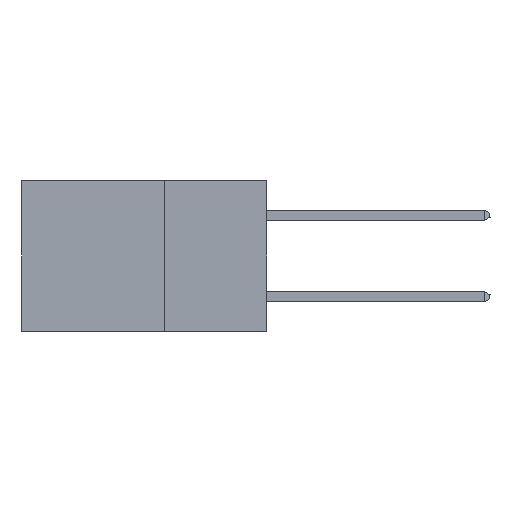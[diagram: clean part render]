
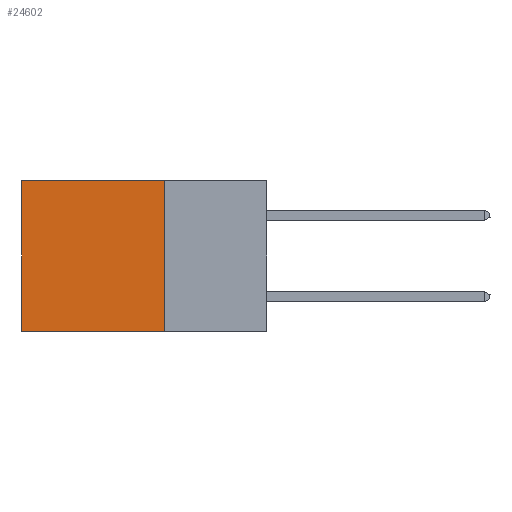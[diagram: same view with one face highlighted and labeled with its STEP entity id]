
A CAD part, left-side view. The second image highlights one B-rep face of the part: STEP entity #24602.
In plain terms, the highlighted planar face has unit normal (-1, 0, 0).
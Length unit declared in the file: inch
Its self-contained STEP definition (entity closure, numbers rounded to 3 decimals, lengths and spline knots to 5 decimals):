
#534 = EDGE_CURVE ( 'NONE', #13739, #16525, #32955, .T. ) ;
#2148 = DIRECTION ( 'NONE',  ( 0., 0., -1. ) ) ;
#2479 = DIRECTION ( 'NONE',  ( 0., 0., -1. ) ) ;
#3390 = DIRECTION ( 'NONE',  ( 0., 1., 0. ) ) ;
#8417 = CARTESIAN_POINT ( 'NONE',  ( 0.2875, 0.6, 0. ) ) ;
#9403 = AXIS2_PLACEMENT_3D ( 'NONE', #19149, #15584, #2479 ) ;
#9864 = EDGE_CURVE ( 'NONE', #23453, #16525, #13088, .T. ) ;
#10249 = CARTESIAN_POINT ( 'NONE',  ( 0.2875, 0.25, 0. ) ) ;
#10642 = VECTOR ( 'NONE', #12633, 39.37008 ) ;
#12633 = DIRECTION ( 'NONE',  ( 0., 1., 0. ) ) ;
#13088 = LINE ( 'NONE', #8417, #23168 ) ;
#13213 = EDGE_LOOP ( 'NONE', ( #23382, #16811, #35172, #29277 ) ) ;
#13739 = VERTEX_POINT ( 'NONE', #31877 ) ;
#14874 = EDGE_CURVE ( 'NONE', #38300, #23453, #29281, .T. ) ;
#15584 = DIRECTION ( 'NONE',  ( 1., 0., 0. ) ) ;
#16525 = VERTEX_POINT ( 'NONE', #26845 ) ;
#16811 = ORIENTED_EDGE ( 'NONE', *, *, #534, .F. ) ;
#19149 = CARTESIAN_POINT ( 'NONE',  ( 0.2875, 0.25, 0. ) ) ;
#21588 = VECTOR ( 'NONE', #22875, 39.37008 ) ;
#22875 = DIRECTION ( 'NONE',  ( 0., 0., -1. ) ) ;
#23168 = VECTOR ( 'NONE', #2148, 39.37008 ) ;
#23382 = ORIENTED_EDGE ( 'NONE', *, *, #9864, .T. ) ;
#23453 = VERTEX_POINT ( 'NONE', #36629 ) ;
#24602 = ADVANCED_FACE ( 'NONE', ( #30479 ), #33254, .F. ) ;
#26845 = CARTESIAN_POINT ( 'NONE',  ( 0.2875, 0.6, -0.37 ) ) ;
#26944 = EDGE_CURVE ( 'NONE', #38300, #13739, #32287, .T. ) ;
#29277 = ORIENTED_EDGE ( 'NONE', *, *, #14874, .T. ) ;
#29281 = LINE ( 'NONE', #40850, #30834 ) ;
#30479 = FACE_OUTER_BOUND ( 'NONE', #13213, .T. ) ;
#30744 = CARTESIAN_POINT ( 'NONE',  ( 0.2875, 0.25, -0.37 ) ) ;
#30834 = VECTOR ( 'NONE', #3390, 39.37008 ) ;
#31877 = CARTESIAN_POINT ( 'NONE',  ( 0.2875, 0.25, -0.37 ) ) ;
#32287 = LINE ( 'NONE', #43262, #21588 ) ;
#32955 = LINE ( 'NONE', #30744, #10642 ) ;
#33254 = PLANE ( 'NONE',  #9403 ) ;
#35172 = ORIENTED_EDGE ( 'NONE', *, *, #26944, .F. ) ;
#36629 = CARTESIAN_POINT ( 'NONE',  ( 0.2875, 0.6, 0. ) ) ;
#38300 = VERTEX_POINT ( 'NONE', #10249 ) ;
#40850 = CARTESIAN_POINT ( 'NONE',  ( 0.2875, 0.25, 0. ) ) ;
#43262 = CARTESIAN_POINT ( 'NONE',  ( 0.2875, 0.25, 0. ) ) ;
